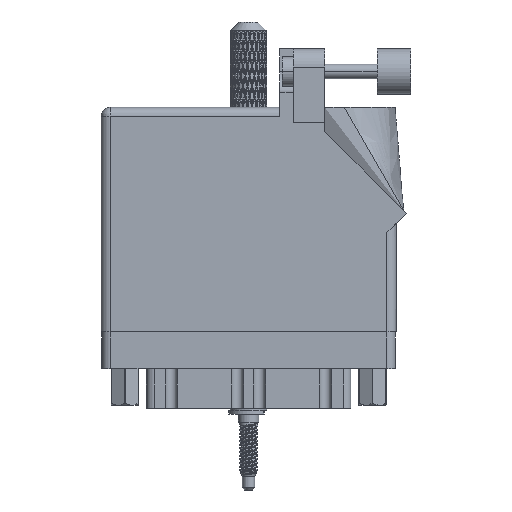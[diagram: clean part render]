
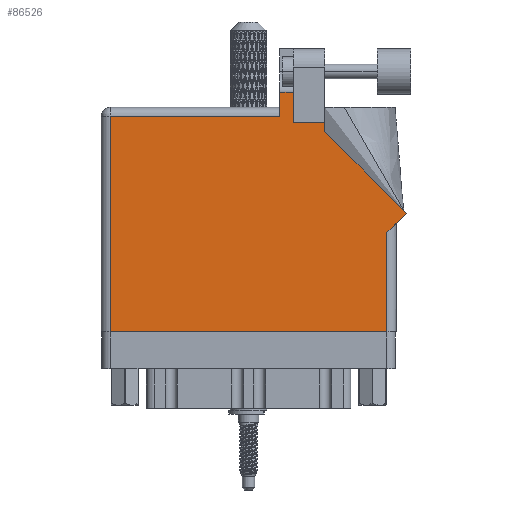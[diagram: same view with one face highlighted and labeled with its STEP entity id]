
A CAD part, front view. The second image highlights one B-rep face of the part: STEP entity #86526.
In plain terms, the highlighted face is planar.
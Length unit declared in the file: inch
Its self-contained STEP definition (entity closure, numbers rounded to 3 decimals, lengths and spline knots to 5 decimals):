
#791 = CARTESIAN_POINT ( 'NONE',  ( 1.311, 1.43, 0. ) ) ;
#2655 = ORIENTED_EDGE ( 'NONE', *, *, #113103, .T. ) ;
#3126 = VERTEX_POINT ( 'NONE', #57391 ) ;
#4722 = CARTESIAN_POINT ( 'NONE',  ( 0., 1.53, 0. ) ) ;
#4917 = EDGE_CURVE ( 'NONE', #93912, #12243, #19128, .T. ) ;
#7026 = LINE ( 'NONE', #102359, #52239 ) ;
#7690 = ORIENTED_EDGE ( 'NONE', *, *, #60184, .T. ) ;
#10377 = CARTESIAN_POINT ( 'NONE',  ( 1.64177, 1.6315, 0. ) ) ;
#12243 = VERTEX_POINT ( 'NONE', #57148 ) ;
#14014 = DIRECTION ( 'NONE',  ( 0., 1., 0. ) ) ;
#14365 = VECTOR ( 'NONE', #19948, 39.37008 ) ;
#15300 = CARTESIAN_POINT ( 'NONE',  ( 0., 1.468, 0. ) ) ;
#15987 = VERTEX_POINT ( 'NONE', #87583 ) ;
#19128 = LINE ( 'NONE', #791, #76457 ) ;
#19735 = EDGE_CURVE ( 'NONE', #59104, #29385, #7026, .T. ) ;
#19948 = DIRECTION ( 'NONE',  ( 0., -1., 0. ) ) ;
#20738 = DIRECTION ( 'NONE',  ( -1., 0., 0. ) ) ;
#21418 = EDGE_CURVE ( 'NONE', #82797, #93912, #83326, .T. ) ;
#21913 = DIRECTION ( 'NONE',  ( 0., 0., -1. ) ) ;
#22734 = ORIENTED_EDGE ( 'NONE', *, *, #76740, .T. ) ;
#27166 = CARTESIAN_POINT ( 'NONE',  ( 1.217, 1.468, 0. ) ) ;
#27172 = DIRECTION ( 'NONE',  ( 0., 1., 0. ) ) ;
#27627 = CARTESIAN_POINT ( 'NONE',  ( 1.524, 1.43, 0. ) ) ;
#27669 = ORIENTED_EDGE ( 'NONE', *, *, #21418, .T. ) ;
#29143 = VECTOR ( 'NONE', #60977, 39.37008 ) ;
#29385 = VERTEX_POINT ( 'NONE', #50256 ) ;
#30073 = ORIENTED_EDGE ( 'NONE', *, *, #84434, .T. ) ;
#31108 = CARTESIAN_POINT ( 'NONE',  ( 0.062, 1.468, 0. ) ) ;
#31402 = EDGE_CURVE ( 'NONE', #35138, #59104, #90998, .T. ) ;
#32033 = CARTESIAN_POINT ( 'NONE',  ( 2.08071, 0.80771, 0. ) ) ;
#32848 = CARTESIAN_POINT ( 'NONE',  ( 0.062, 0., 0. ) ) ;
#33227 = VECTOR ( 'NONE', #77325, 39.37008 ) ;
#35138 = VERTEX_POINT ( 'NONE', #111657 ) ;
#36239 = ORIENTED_EDGE ( 'NONE', *, *, #4917, .T. ) ;
#39292 = LINE ( 'NONE', #74334, #63823 ) ;
#39727 = EDGE_CURVE ( 'NONE', #88309, #60923, #85115, .T. ) ;
#41208 = DIRECTION ( 'NONE',  ( -0.707, 0.707, 0. ) ) ;
#42040 = DIRECTION ( 'NONE',  ( 0.707, 0.707, 0. ) ) ;
#46643 = FACE_OUTER_BOUND ( 'NONE', #95653, .T. ) ;
#48862 = CARTESIAN_POINT ( 'NONE',  ( 1.524, 1.43, 0. ) ) ;
#48918 = DIRECTION ( 'NONE',  ( -1., 0., 0. ) ) ;
#49265 = LINE ( 'NONE', #32033, #103151 ) ;
#49679 = CARTESIAN_POINT ( 'NONE',  ( 1.311, 1.43, 0. ) ) ;
#50256 = CARTESIAN_POINT ( 'NONE',  ( 2.08071, 0.80771, 0. ) ) ;
#51766 = CARTESIAN_POINT ( 'NONE',  ( 0., 0., 0. ) ) ;
#52239 = VECTOR ( 'NONE', #42040, 39.37008 ) ;
#57148 = CARTESIAN_POINT ( 'NONE',  ( 1.311, 1.6315, 0. ) ) ;
#57391 = CARTESIAN_POINT ( 'NONE',  ( 1.524, 1.36442, 0. ) ) ;
#59104 = VERTEX_POINT ( 'NONE', #108095 ) ;
#59832 = VECTOR ( 'NONE', #20738, 39.37008 ) ;
#60184 = EDGE_CURVE ( 'NONE', #60923, #35138, #87375, .T. ) ;
#60923 = VERTEX_POINT ( 'NONE', #107580 ) ;
#60977 = DIRECTION ( 'NONE',  ( 1., 0., 0. ) ) ;
#61362 = ORIENTED_EDGE ( 'NONE', *, *, #31402, .T. ) ;
#63221 = LINE ( 'NONE', #10377, #112494 ) ;
#63823 = VECTOR ( 'NONE', #14014, 39.37008 ) ;
#68492 = AXIS2_PLACEMENT_3D ( 'NONE', #4722, #21913, #48918 ) ;
#74334 = CARTESIAN_POINT ( 'NONE',  ( 1.524, 1.36442, 0. ) ) ;
#76457 = VECTOR ( 'NONE', #27172, 39.37008 ) ;
#76740 = EDGE_CURVE ( 'NONE', #77299, #88309, #94566, .T. ) ;
#77299 = VERTEX_POINT ( 'NONE', #27166 ) ;
#77325 = DIRECTION ( 'NONE',  ( -1., 0., 0. ) ) ;
#77865 = VECTOR ( 'NONE', #102943, 39.37008 ) ;
#79391 = ORIENTED_EDGE ( 'NONE', *, *, #39727, .T. ) ;
#82258 = PLANE ( 'NONE',  #68492 ) ;
#82383 = DIRECTION ( 'NONE',  ( 0., 1., 0. ) ) ;
#82797 = VERTEX_POINT ( 'NONE', #27627 ) ;
#83326 = LINE ( 'NONE', #48862, #59832 ) ;
#84434 = EDGE_CURVE ( 'NONE', #29385, #3126, #49265, .T. ) ;
#85115 = LINE ( 'NONE', #32848, #77865 ) ;
#86526 = ADVANCED_FACE ( 'NONE', ( #46643 ), #82258, .F. ) ;
#87375 = LINE ( 'NONE', #51766, #29143 ) ;
#87480 = EDGE_CURVE ( 'NONE', #12243, #15987, #63221, .T. ) ;
#87583 = CARTESIAN_POINT ( 'NONE',  ( 1.217, 1.6315, 0. ) ) ;
#88309 = VERTEX_POINT ( 'NONE', #31108 ) ;
#88488 = DIRECTION ( 'NONE',  ( -1., 0., 0. ) ) ;
#90998 = LINE ( 'NONE', #92123, #92531 ) ;
#91035 = ORIENTED_EDGE ( 'NONE', *, *, #87480, .T. ) ;
#92123 = CARTESIAN_POINT ( 'NONE',  ( 1.948, 0.737, 0. ) ) ;
#92531 = VECTOR ( 'NONE', #82383, 39.37008 ) ;
#93912 = VERTEX_POINT ( 'NONE', #49679 ) ;
#94566 = LINE ( 'NONE', #15300, #33227 ) ;
#95653 = EDGE_LOOP ( 'NONE', ( #36239, #91035, #110269, #22734, #79391, #7690, #61362, #97268, #30073, #2655, #27669 ) ) ;
#97268 = ORIENTED_EDGE ( 'NONE', *, *, #19735, .T. ) ;
#102359 = CARTESIAN_POINT ( 'NONE',  ( 2.01, 0.737, 0. ) ) ;
#102943 = DIRECTION ( 'NONE',  ( 0., -1., 0. ) ) ;
#103151 = VECTOR ( 'NONE', #41208, 39.37008 ) ;
#107242 = LINE ( 'NONE', #107806, #14365 ) ;
#107580 = CARTESIAN_POINT ( 'NONE',  ( 0.062, 0., 0. ) ) ;
#107806 = CARTESIAN_POINT ( 'NONE',  ( 1.217, 1.53, 0. ) ) ;
#108095 = CARTESIAN_POINT ( 'NONE',  ( 1.948, 0.675, 0. ) ) ;
#110269 = ORIENTED_EDGE ( 'NONE', *, *, #113591, .T. ) ;
#111657 = CARTESIAN_POINT ( 'NONE',  ( 1.948, 0., 0. ) ) ;
#112494 = VECTOR ( 'NONE', #88488, 39.37008 ) ;
#113103 = EDGE_CURVE ( 'NONE', #3126, #82797, #39292, .T. ) ;
#113591 = EDGE_CURVE ( 'NONE', #15987, #77299, #107242, .T. ) ;
